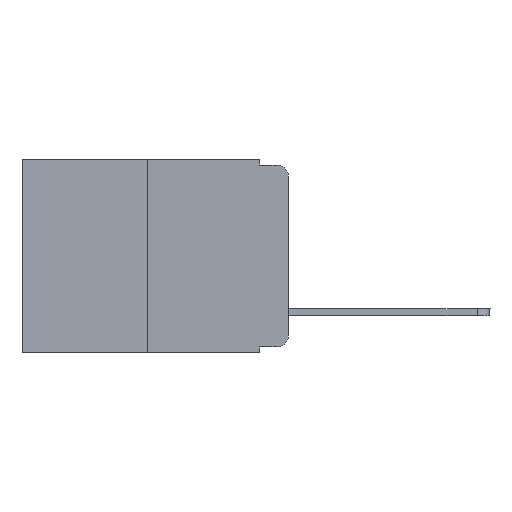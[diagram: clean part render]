
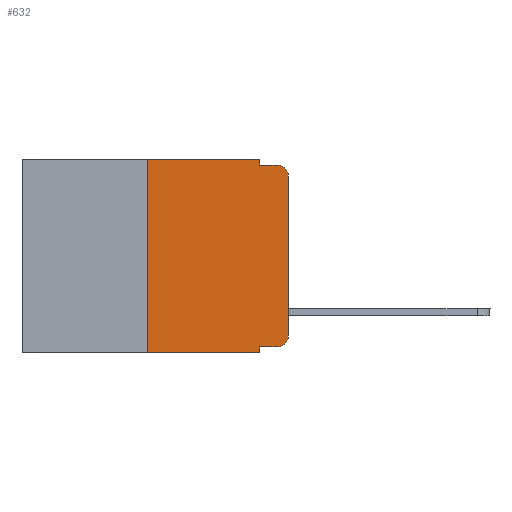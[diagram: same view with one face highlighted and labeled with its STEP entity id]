
A CAD part, left-side view. The second image highlights one B-rep face of the part: STEP entity #632.
In plain terms, the highlighted planar face has unit normal (-1, 0, 0).
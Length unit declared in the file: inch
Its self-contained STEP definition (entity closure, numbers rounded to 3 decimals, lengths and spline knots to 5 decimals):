
#18 = ORIENTED_EDGE ( 'NONE', *, *, #1689, .T. ) ;
#174 = LINE ( 'NONE', #10970, #4427 ) ;
#386 = ORIENTED_EDGE ( 'NONE', *, *, #7669, .T. ) ;
#388 = EDGE_CURVE ( 'NONE', #4531, #9850, #1300, .T. ) ;
#395 = DIRECTION ( 'NONE',  ( 0., 0., -1. ) ) ;
#481 = FACE_OUTER_BOUND ( 'NONE', #5478, .T. ) ;
#556 = CARTESIAN_POINT ( 'NONE',  ( 0., 0.02, -0.313 ) ) ;
#632 = ADVANCED_FACE ( 'NONE', ( #481 ), #9921, .F. ) ;
#1300 = LINE ( 'NONE', #1740, #3770 ) ;
#1336 = VERTEX_POINT ( 'NONE', #3152 ) ;
#1689 = EDGE_CURVE ( 'NONE', #6491, #6706, #2215, .T. ) ;
#1701 = CARTESIAN_POINT ( 'NONE',  ( 0., 0.051, 0. ) ) ;
#1740 = CARTESIAN_POINT ( 'NONE',  ( 0., 0.051, 0. ) ) ;
#2023 = CARTESIAN_POINT ( 'NONE',  ( 0., 0.25, -0.343 ) ) ;
#2215 = LINE ( 'NONE', #5653, #3605 ) ;
#2233 = CARTESIAN_POINT ( 'NONE',  ( 0., 0.02, -0.333 ) ) ;
#2696 = EDGE_CURVE ( 'NONE', #3206, #5519, #4815, .T. ) ;
#2724 = ORIENTED_EDGE ( 'NONE', *, *, #9258, .F. ) ;
#2780 = CARTESIAN_POINT ( 'NONE',  ( 0., 0.02, -0.01 ) ) ;
#2818 = VECTOR ( 'NONE', #9763, 39.37008 ) ;
#3088 = LINE ( 'NONE', #3594, #2818 ) ;
#3152 = CARTESIAN_POINT ( 'NONE',  ( 0., 0., -0.03 ) ) ;
#3206 = VERTEX_POINT ( 'NONE', #9165 ) ;
#3249 = LINE ( 'NONE', #8643, #5330 ) ;
#3320 = DIRECTION ( 'NONE',  ( 0., 0., -1. ) ) ;
#3594 = CARTESIAN_POINT ( 'NONE',  ( 0., 0.473, 0. ) ) ;
#3605 = VECTOR ( 'NONE', #10103, 39.37008 ) ;
#3665 = VECTOR ( 'NONE', #6393, 39.37008 ) ;
#3770 = VECTOR ( 'NONE', #3320, 39.37008 ) ;
#4166 = ORIENTED_EDGE ( 'NONE', *, *, #11153, .F. ) ;
#4424 = VERTEX_POINT ( 'NONE', #2780 ) ;
#4427 = VECTOR ( 'NONE', #4857, 39.37008 ) ;
#4531 = VERTEX_POINT ( 'NONE', #9132 ) ;
#4615 = EDGE_CURVE ( 'NONE', #6491, #10305, #174, .T. ) ;
#4815 = LINE ( 'NONE', #11172, #11184 ) ;
#4857 = DIRECTION ( 'NONE',  ( 0., 0., 1. ) ) ;
#5066 = ORIENTED_EDGE ( 'NONE', *, *, #2696, .T. ) ;
#5078 = DIRECTION ( 'NONE',  ( 0., 0., -1. ) ) ;
#5330 = VECTOR ( 'NONE', #9648, 39.37008 ) ;
#5446 = AXIS2_PLACEMENT_3D ( 'NONE', #9181, #10048, #395 ) ;
#5467 = EDGE_CURVE ( 'NONE', #5519, #6345, #11180, .T. ) ;
#5478 = EDGE_LOOP ( 'NONE', ( #8890, #386, #2724, #6318, #4166, #8775, #18, #8530, #5066, #10164 ) ) ;
#5519 = VERTEX_POINT ( 'NONE', #2233 ) ;
#5653 = CARTESIAN_POINT ( 'NONE',  ( 0., 0.473, -0.343 ) ) ;
#5719 = DIRECTION ( 'NONE',  ( 0., -1., 0. ) ) ;
#5778 = DIRECTION ( 'NONE',  ( 0., 0., -1. ) ) ;
#6318 = ORIENTED_EDGE ( 'NONE', *, *, #388, .F. ) ;
#6345 = VERTEX_POINT ( 'NONE', #10160 ) ;
#6393 = DIRECTION ( 'NONE',  ( 0., 0., 1. ) ) ;
#6403 = DIRECTION ( 'NONE',  ( 0., 0., -1. ) ) ;
#6491 = VERTEX_POINT ( 'NONE', #2023 ) ;
#6706 = VERTEX_POINT ( 'NONE', #8948 ) ;
#7456 = DIRECTION ( 'NONE',  ( -1., 0., 0. ) ) ;
#7669 = EDGE_CURVE ( 'NONE', #1336, #4424, #9853, .T. ) ;
#8070 = CARTESIAN_POINT ( 'NONE',  ( 0., 0., 0. ) ) ;
#8530 = ORIENTED_EDGE ( 'NONE', *, *, #10997, .F. ) ;
#8643 = CARTESIAN_POINT ( 'NONE',  ( 0., 0.051, -0.01 ) ) ;
#8775 = ORIENTED_EDGE ( 'NONE', *, *, #4615, .F. ) ;
#8881 = LINE ( 'NONE', #8070, #3665 ) ;
#8890 = ORIENTED_EDGE ( 'NONE', *, *, #11292, .T. ) ;
#8948 = CARTESIAN_POINT ( 'NONE',  ( 0., 0.051, -0.343 ) ) ;
#9029 = CARTESIAN_POINT ( 'NONE',  ( 0., 0.02, -0.03 ) ) ;
#9132 = CARTESIAN_POINT ( 'NONE',  ( 0., 0.051, 0. ) ) ;
#9165 = CARTESIAN_POINT ( 'NONE',  ( 0., 0.051, -0.333 ) ) ;
#9181 = CARTESIAN_POINT ( 'NONE',  ( 0., 0.473, 0. ) ) ;
#9258 = EDGE_CURVE ( 'NONE', #9850, #4424, #3249, .T. ) ;
#9393 = CARTESIAN_POINT ( 'NONE',  ( 0., 0.25, 0. ) ) ;
#9648 = DIRECTION ( 'NONE',  ( 0., -1., 0. ) ) ;
#9763 = DIRECTION ( 'NONE',  ( 0., -1., 0. ) ) ;
#9838 = AXIS2_PLACEMENT_3D ( 'NONE', #9029, #10825, #6403 ) ;
#9850 = VERTEX_POINT ( 'NONE', #11240 ) ;
#9853 = CIRCLE ( 'NONE', #9838, 0.02 ) ;
#9921 = PLANE ( 'NONE',  #5446 ) ;
#10048 = DIRECTION ( 'NONE',  ( 1., 0., 0. ) ) ;
#10103 = DIRECTION ( 'NONE',  ( 0., -1., 0. ) ) ;
#10159 = LINE ( 'NONE', #1701, #11125 ) ;
#10160 = CARTESIAN_POINT ( 'NONE',  ( 0., 0., -0.313 ) ) ;
#10164 = ORIENTED_EDGE ( 'NONE', *, *, #5467, .T. ) ;
#10305 = VERTEX_POINT ( 'NONE', #9393 ) ;
#10825 = DIRECTION ( 'NONE',  ( -1., 0., 0. ) ) ;
#10970 = CARTESIAN_POINT ( 'NONE',  ( 0., 0.25, 0. ) ) ;
#10997 = EDGE_CURVE ( 'NONE', #3206, #6706, #10159, .T. ) ;
#11003 = AXIS2_PLACEMENT_3D ( 'NONE', #556, #7456, #5778 ) ;
#11125 = VECTOR ( 'NONE', #5078, 39.37008 ) ;
#11153 = EDGE_CURVE ( 'NONE', #10305, #4531, #3088, .T. ) ;
#11172 = CARTESIAN_POINT ( 'NONE',  ( 0., 0.051, -0.333 ) ) ;
#11180 = CIRCLE ( 'NONE', #11003, 0.02 ) ;
#11184 = VECTOR ( 'NONE', #5719, 39.37008 ) ;
#11240 = CARTESIAN_POINT ( 'NONE',  ( 0., 0.051, -0.01 ) ) ;
#11292 = EDGE_CURVE ( 'NONE', #6345, #1336, #8881, .T. ) ;
